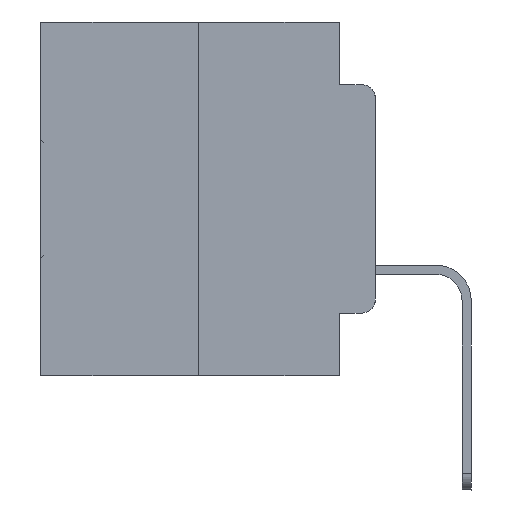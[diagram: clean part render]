
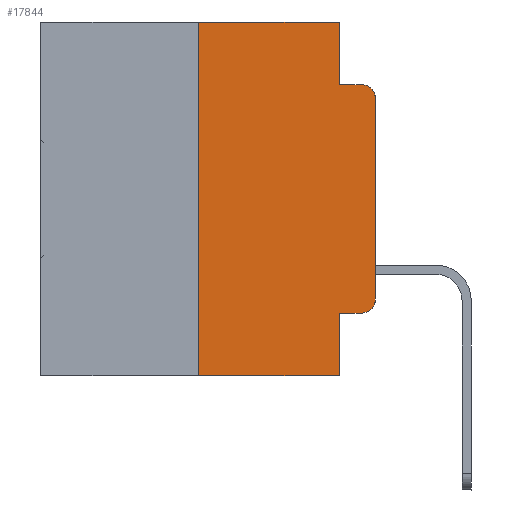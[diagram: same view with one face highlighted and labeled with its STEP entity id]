
A CAD part, left-side view. The second image highlights one B-rep face of the part: STEP entity #17844.
In plain terms, the highlighted planar face has unit normal (-1, 0, 0).
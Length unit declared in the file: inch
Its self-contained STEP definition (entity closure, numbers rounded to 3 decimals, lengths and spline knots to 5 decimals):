
#415 = EDGE_CURVE ( 'NONE', #15470, #29969, #10575, .T. ) ;
#533 = LINE ( 'NONE', #9250, #30045 ) ;
#1200 = CARTESIAN_POINT ( 'NONE',  ( 0., 0.02, -0.0885 ) ) ;
#1471 = DIRECTION ( 'NONE',  ( 0., 0., -1. ) ) ;
#1962 = CARTESIAN_POINT ( 'NONE',  ( 0., 0.051, -0.0885 ) ) ;
#3901 = CIRCLE ( 'NONE', #28991, 0.02 ) ;
#3951 = CIRCLE ( 'NONE', #15215, 0.02 ) ;
#4031 = VECTOR ( 'NONE', #26420, 39.37008 ) ;
#4075 = ORIENTED_EDGE ( 'NONE', *, *, #20367, .F. ) ;
#4122 = VERTEX_POINT ( 'NONE', #12613 ) ;
#4456 = VECTOR ( 'NONE', #9640, 39.37008 ) ;
#4459 = DIRECTION ( 'NONE',  ( 0., -1., 0. ) ) ;
#4613 = ORIENTED_EDGE ( 'NONE', *, *, #24033, .T. ) ;
#5835 = LINE ( 'NONE', #25509, #24152 ) ;
#5946 = EDGE_CURVE ( 'NONE', #6944, #4122, #25922, .T. ) ;
#6121 = VERTEX_POINT ( 'NONE', #1200 ) ;
#6670 = VERTEX_POINT ( 'NONE', #17769 ) ;
#6865 = DIRECTION ( 'NONE',  ( -1., 0., 0. ) ) ;
#6944 = VERTEX_POINT ( 'NONE', #23717 ) ;
#7240 = CARTESIAN_POINT ( 'NONE',  ( 0., 0.051, -0.4115 ) ) ;
#9172 = CARTESIAN_POINT ( 'NONE',  ( 0., 0.02, -0.3915 ) ) ;
#9250 = CARTESIAN_POINT ( 'NONE',  ( 0., 0.051, 0. ) ) ;
#9265 = CARTESIAN_POINT ( 'NONE',  ( 0., 0.02, -0.1085 ) ) ;
#9640 = DIRECTION ( 'NONE',  ( 0., 0., 1. ) ) ;
#9894 = VECTOR ( 'NONE', #4459, 39.37008 ) ;
#9961 = CARTESIAN_POINT ( 'NONE',  ( 0., 0., -0.1085 ) ) ;
#10575 = LINE ( 'NONE', #12490, #27725 ) ;
#10680 = ORIENTED_EDGE ( 'NONE', *, *, #28707, .T. ) ;
#11350 = EDGE_CURVE ( 'NONE', #4122, #26994, #533, .T. ) ;
#11419 = CARTESIAN_POINT ( 'NONE',  ( 0., 0.25, 0. ) ) ;
#11624 = DIRECTION ( 'NONE',  ( 1., 0., 0. ) ) ;
#12490 = CARTESIAN_POINT ( 'NONE',  ( 0., 0.473, -0.5 ) ) ;
#12613 = CARTESIAN_POINT ( 'NONE',  ( 0., 0.051, 0. ) ) ;
#13850 = ORIENTED_EDGE ( 'NONE', *, *, #29284, .F. ) ;
#13881 = DIRECTION ( 'NONE',  ( -1., 0., 0. ) ) ;
#14046 = EDGE_CURVE ( 'NONE', #19038, #14433, #3901, .T. ) ;
#14145 = CARTESIAN_POINT ( 'NONE',  ( 0., 0.051, -0.5 ) ) ;
#14433 = VERTEX_POINT ( 'NONE', #22505 ) ;
#15123 = EDGE_CURVE ( 'NONE', #14433, #30087, #21791, .T. ) ;
#15215 = AXIS2_PLACEMENT_3D ( 'NONE', #9265, #6865, #25947 ) ;
#15246 = ORIENTED_EDGE ( 'NONE', *, *, #11350, .F. ) ;
#15470 = VERTEX_POINT ( 'NONE', #28784 ) ;
#16253 = DIRECTION ( 'NONE',  ( 0., 0., -1. ) ) ;
#16766 = LINE ( 'NONE', #7240, #4031 ) ;
#17769 = CARTESIAN_POINT ( 'NONE',  ( 0., 0.051, -0.4115 ) ) ;
#17844 = ADVANCED_FACE ( 'NONE', ( #26843 ), #18483, .F. ) ;
#18060 = CARTESIAN_POINT ( 'NONE',  ( 0., 0., 0. ) ) ;
#18483 = PLANE ( 'NONE',  #23470 ) ;
#18612 = ORIENTED_EDGE ( 'NONE', *, *, #27089, .F. ) ;
#19038 = VERTEX_POINT ( 'NONE', #25521 ) ;
#19584 = VECTOR ( 'NONE', #26703, 39.37008 ) ;
#20367 = EDGE_CURVE ( 'NONE', #26994, #6121, #29631, .T. ) ;
#20651 = VECTOR ( 'NONE', #27352, 39.37008 ) ;
#20844 = ORIENTED_EDGE ( 'NONE', *, *, #15123, .T. ) ;
#20888 = DIRECTION ( 'NONE',  ( 0., 0., -1. ) ) ;
#21791 = LINE ( 'NONE', #18060, #20651 ) ;
#21808 = CARTESIAN_POINT ( 'NONE',  ( 0., 0.473, 0. ) ) ;
#22505 = CARTESIAN_POINT ( 'NONE',  ( 0., 0., -0.3915 ) ) ;
#23349 = DIRECTION ( 'NONE',  ( 0., 0., -1. ) ) ;
#23470 = AXIS2_PLACEMENT_3D ( 'NONE', #30365, #11624, #20888 ) ;
#23536 = LINE ( 'NONE', #11419, #4456 ) ;
#23717 = CARTESIAN_POINT ( 'NONE',  ( 0., 0.25, 0. ) ) ;
#24033 = EDGE_CURVE ( 'NONE', #6670, #19038, #16766, .T. ) ;
#24124 = ORIENTED_EDGE ( 'NONE', *, *, #14046, .T. ) ;
#24152 = VECTOR ( 'NONE', #1471, 39.37008 ) ;
#25284 = ORIENTED_EDGE ( 'NONE', *, *, #415, .T. ) ;
#25509 = CARTESIAN_POINT ( 'NONE',  ( 0., 0.051, 0. ) ) ;
#25521 = CARTESIAN_POINT ( 'NONE',  ( 0., 0.02, -0.4115 ) ) ;
#25922 = LINE ( 'NONE', #21808, #19584 ) ;
#25947 = DIRECTION ( 'NONE',  ( 0., 0., -1. ) ) ;
#26086 = CARTESIAN_POINT ( 'NONE',  ( 0., 0.051, -0.0885 ) ) ;
#26420 = DIRECTION ( 'NONE',  ( 0., -1., 0. ) ) ;
#26703 = DIRECTION ( 'NONE',  ( 0., -1., 0. ) ) ;
#26736 = ORIENTED_EDGE ( 'NONE', *, *, #5946, .F. ) ;
#26843 = FACE_OUTER_BOUND ( 'NONE', #28734, .T. ) ;
#26994 = VERTEX_POINT ( 'NONE', #1962 ) ;
#27089 = EDGE_CURVE ( 'NONE', #15470, #6944, #23536, .T. ) ;
#27352 = DIRECTION ( 'NONE',  ( 0., 0., 1. ) ) ;
#27725 = VECTOR ( 'NONE', #29144, 39.37008 ) ;
#28707 = EDGE_CURVE ( 'NONE', #30087, #6121, #3951, .T. ) ;
#28734 = EDGE_LOOP ( 'NONE', ( #20844, #10680, #4075, #15246, #26736, #18612, #25284, #13850, #4613, #24124 ) ) ;
#28784 = CARTESIAN_POINT ( 'NONE',  ( 0., 0.25, -0.5 ) ) ;
#28991 = AXIS2_PLACEMENT_3D ( 'NONE', #9172, #13881, #23349 ) ;
#29144 = DIRECTION ( 'NONE',  ( 0., -1., 0. ) ) ;
#29284 = EDGE_CURVE ( 'NONE', #6670, #29969, #5835, .T. ) ;
#29631 = LINE ( 'NONE', #26086, #9894 ) ;
#29969 = VERTEX_POINT ( 'NONE', #14145 ) ;
#30045 = VECTOR ( 'NONE', #16253, 39.37008 ) ;
#30087 = VERTEX_POINT ( 'NONE', #9961 ) ;
#30365 = CARTESIAN_POINT ( 'NONE',  ( 0., 0.473, 0. ) ) ;
